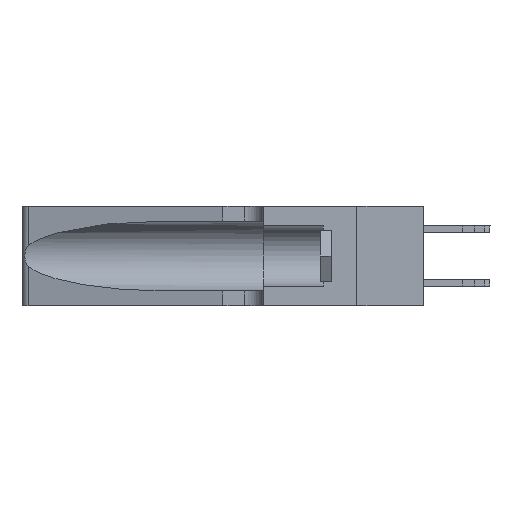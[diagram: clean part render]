
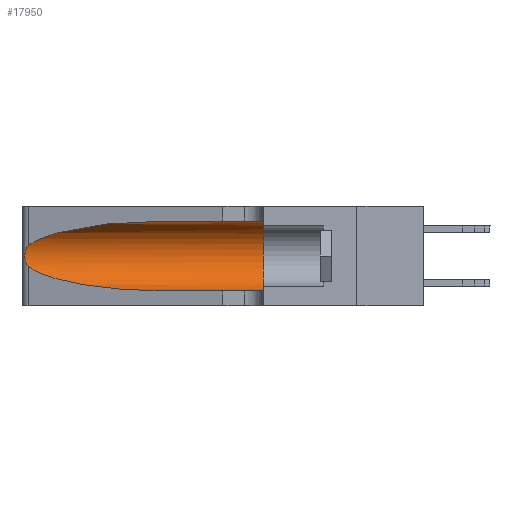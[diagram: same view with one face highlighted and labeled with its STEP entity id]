
A CAD part, left-side view. The second image highlights one B-rep face of the part: STEP entity #17950.
In plain terms, the highlighted cylindrical face has radius 3.308 mm (diameter 6.617 mm), a partial arc.
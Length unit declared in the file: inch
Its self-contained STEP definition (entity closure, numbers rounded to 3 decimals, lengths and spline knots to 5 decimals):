
#172 = CARTESIAN_POINT ( 'NONE',  ( 0.25487, 1.22718, 0.22369 ) ) ;
#787 = CARTESIAN_POINT ( 'NONE',  ( 0.1305, 1.61858, 0.185 ) ) ;
#985 = EDGE_CURVE ( 'NONE', #30541, #12647, #2491, .T. ) ;
#1078 = VERTEX_POINT ( 'NONE', #4681 ) ;
#1727 = CARTESIAN_POINT ( 'NONE',  ( 0.18966, 0.96281, 0.31525 ) ) ;
#1900 = EDGE_LOOP ( 'NONE', ( #20781, #26626, #30182, #24599, #2671, #3913 ) ) ;
#1980 = VECTOR ( 'NONE', #22702, 39.37008 ) ;
#2491 = B_SPLINE_CURVE_WITH_KNOTS ( 'NONE', 3,
 ( #26473, #31280, #21295, #28941, #26580, #11422, #11532, #14364, #28730, #11755, #31383, #6918, #18745, #16708 ),
 .UNSPECIFIED., .F., .F.,
 ( 4, 2, 2, 2, 2, 2, 4 ),
 ( 0., 0.00027, 0.00053, 0.00107, 0.0016, 0.00187, 0.00214 ),
 .UNSPECIFIED. ) ;
#2671 = ORIENTED_EDGE ( 'NONE', *, *, #4890, .F. ) ;
#2681 = CARTESIAN_POINT ( 'NONE',  ( 0.1305, 0.35, 0.31525 ) ) ;
#2859 = DIRECTION ( 'NONE',  ( 0., -1., 0. ) ) ;
#3913 = ORIENTED_EDGE ( 'NONE', *, *, #13751, .F. ) ;
#4681 = CARTESIAN_POINT ( 'NONE',  ( 0.1305, 0.72297, 0.31525 ) ) ;
#4742 = DIRECTION ( 'NONE',  ( 0., 1., 0. ) ) ;
#4890 = EDGE_CURVE ( 'NONE', #28633, #24671, #26684, .T. ) ;
#5950 = DIRECTION ( 'NONE',  ( 0., -1., 0. ) ) ;
#6617 = VECTOR ( 'NONE', #2859, 39.37008 ) ;
#6918 = CARTESIAN_POINT ( 'NONE',  ( 0.25639, 1.23186, 0.15144 ) ) ;
#7088 = EDGE_CURVE ( 'NONE', #1078, #30541, #16870, .T. ) ;
#8790 = VERTEX_POINT ( 'NONE', #28738 ) ;
#10475 = EDGE_CURVE ( 'NONE', #12647, #8790, #27824, .T. ) ;
#10751 = CARTESIAN_POINT ( 'NONE',  ( 0.1305, 0.72297, 0.05475 ) ) ;
#11422 = CARTESIAN_POINT ( 'NONE',  ( 0.26018, 1.23835, 0.19895 ) ) ;
#11532 = CARTESIAN_POINT ( 'NONE',  ( 0.26075, 1.23896, 0.19203 ) ) ;
#11726 = CARTESIAN_POINT ( 'NONE',  ( 0.1305, 1.61858, 0.31525 ) ) ;
#11755 = CARTESIAN_POINT ( 'NONE',  ( 0.25856, 1.23593, 0.16098 ) ) ;
#12647 = VERTEX_POINT ( 'NONE', #26906 ) ;
#13751 = EDGE_CURVE ( 'NONE', #1078, #28633, #23490, .T. ) ;
#14109 = FACE_OUTER_BOUND ( 'NONE', #1900, .T. ) ;
#14310 = LINE ( 'NONE', #24762, #1980 ) ;
#14364 = CARTESIAN_POINT ( 'NONE',  ( 0.26075, 1.23896, 0.178 ) ) ;
#16400 = AXIS2_PLACEMENT_3D ( 'NONE', #19478, #4742, #21908 ) ;
#16708 = CARTESIAN_POINT ( 'NONE',  ( 0.25487, 1.22718, 0.14631 ) ) ;
#16870 =( BOUNDED_CURVE ( )  B_SPLINE_CURVE ( 3, ( #21777, #1727, #17204, #172 ),
 .UNSPECIFIED., .F., .F. ) 
 B_SPLINE_CURVE_WITH_KNOTS ( ( 4, 4 ),
 ( 1.5708, 2.84003 ),
 .UNSPECIFIED. ) 
 CURVE ( )  GEOMETRIC_REPRESENTATION_ITEM ( )  RATIONAL_B_SPLINE_CURVE ( ( 1., 0.87, 0.87, 1. ) ) 
 REPRESENTATION_ITEM ( '' )  );
#17204 = CARTESIAN_POINT ( 'NONE',  ( 0.2373, 1.15595, 0.28018 ) ) ;
#17415 = CARTESIAN_POINT ( 'NONE',  ( 0.25487, 1.22718, 0.22369 ) ) ;
#17950 = ADVANCED_FACE ( 'NONE', ( #14109 ), #31348, .F. ) ;
#18745 = CARTESIAN_POINT ( 'NONE',  ( 0.25555, 1.22993, 0.14849 ) ) ;
#19478 = CARTESIAN_POINT ( 'NONE',  ( 0.1305, 0.35, 0.185 ) ) ;
#20781 = ORIENTED_EDGE ( 'NONE', *, *, #7088, .T. ) ;
#20946 = EDGE_CURVE ( 'NONE', #8790, #24671, #14310, .T. ) ;
#21295 = CARTESIAN_POINT ( 'NONE',  ( 0.25639, 1.23184, 0.21858 ) ) ;
#21638 = CARTESIAN_POINT ( 'NONE',  ( 0.25487, 1.22718, 0.14631 ) ) ;
#21777 = CARTESIAN_POINT ( 'NONE',  ( 0.1305, 0.72297, 0.31525 ) ) ;
#21908 = DIRECTION ( 'NONE',  ( 0., 0., 1. ) ) ;
#22455 = CARTESIAN_POINT ( 'NONE',  ( 0.2373, 1.15595, 0.08982 ) ) ;
#22702 = DIRECTION ( 'NONE',  ( 0., -1., 0. ) ) ;
#22873 = CARTESIAN_POINT ( 'NONE',  ( 0.18966, 0.96281, 0.05475 ) ) ;
#23013 = DIRECTION ( 'NONE',  ( 0., 0., -1. ) ) ;
#23490 = LINE ( 'NONE', #11726, #6617 ) ;
#24238 = CARTESIAN_POINT ( 'NONE',  ( 0.1305, 0.35, 0.05475 ) ) ;
#24599 = ORIENTED_EDGE ( 'NONE', *, *, #20946, .T. ) ;
#24671 = VERTEX_POINT ( 'NONE', #24238 ) ;
#24762 = CARTESIAN_POINT ( 'NONE',  ( 0.1305, 1.61858, 0.05475 ) ) ;
#26473 = CARTESIAN_POINT ( 'NONE',  ( 0.25487, 1.22718, 0.22369 ) ) ;
#26580 = CARTESIAN_POINT ( 'NONE',  ( 0.25854, 1.2359, 0.20912 ) ) ;
#26626 = ORIENTED_EDGE ( 'NONE', *, *, #985, .T. ) ;
#26684 = CIRCLE ( 'NONE', #16400, 0.13025 ) ;
#26906 = CARTESIAN_POINT ( 'NONE',  ( 0.25487, 1.22718, 0.14631 ) ) ;
#27824 =( BOUNDED_CURVE ( )  B_SPLINE_CURVE ( 3, ( #21638, #22455, #22873, #10751 ),
 .UNSPECIFIED., .F., .F. ) 
 B_SPLINE_CURVE_WITH_KNOTS ( ( 4, 4 ),
 ( 3.44316, 4.71239 ),
 .UNSPECIFIED. ) 
 CURVE ( )  GEOMETRIC_REPRESENTATION_ITEM ( )  RATIONAL_B_SPLINE_CURVE ( ( 1., 0.87, 0.87, 1. ) ) 
 REPRESENTATION_ITEM ( '' )  );
#28633 = VERTEX_POINT ( 'NONE', #2681 ) ;
#28730 = CARTESIAN_POINT ( 'NONE',  ( 0.26017, 1.23833, 0.17102 ) ) ;
#28738 = CARTESIAN_POINT ( 'NONE',  ( 0.1305, 0.72297, 0.05475 ) ) ;
#28941 = CARTESIAN_POINT ( 'NONE',  ( 0.25787, 1.23484, 0.2124 ) ) ;
#30182 = ORIENTED_EDGE ( 'NONE', *, *, #10475, .T. ) ;
#30541 = VERTEX_POINT ( 'NONE', #17415 ) ;
#31280 = CARTESIAN_POINT ( 'NONE',  ( 0.25555, 1.22994, 0.2215 ) ) ;
#31348 = CYLINDRICAL_SURFACE ( 'NONE', #31475, 0.13025 ) ;
#31383 = CARTESIAN_POINT ( 'NONE',  ( 0.25789, 1.23486, 0.15765 ) ) ;
#31475 = AXIS2_PLACEMENT_3D ( 'NONE', #787, #5950, #23013 ) ;
